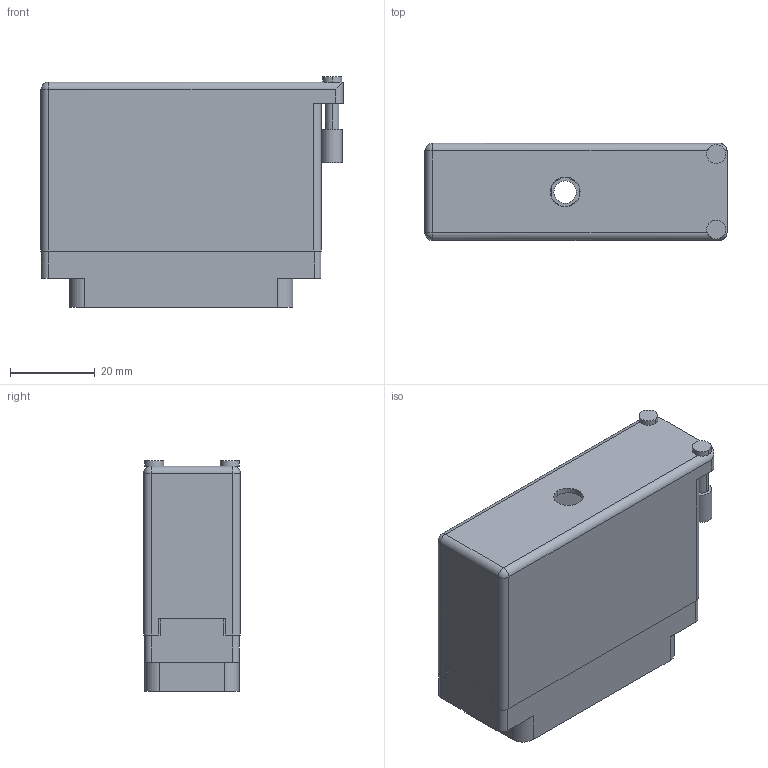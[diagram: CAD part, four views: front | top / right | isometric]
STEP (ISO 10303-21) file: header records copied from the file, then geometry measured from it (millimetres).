
FILE_DESCRIPTION (( 'STEP AP203' ), '1' );
FILE_NAME ('516-056-000-150.STEP', '2020-03-10T04:10:37', ( '' ), ( '' ), 'SwSTEP 2.0', 'SolidWorks 2016', '' );
FILE_SCHEMA (( 'CONFIG_CONTROL_DESIGN' ));
Length unit declared in the file: inch
Products named in the file (3): 516-056-000-150; 516 Plug Insulator_056; 516-230-001_Metal - 056 Side Entry
Assembly tree (2 placements, depth 2):
  516-056-000-150
    516 Plug Insulator_056
    516-230-001_Metal - 056 Side Entry
Bounding box: 71.12 x 22.83 x 54.31 mm (x, y, z)
Volume: 21855.5 mm3; surface area: 31798.8 mm2
Topology: 2 solids, 2 shells, 1280 faces, 3763 edges, 2502 vertices
Faces by surface type: plane 930, cylinder 346, cone 2, sphere 2
Entity records: 43134 total; most frequent: CARTESIAN_POINT 7589, ORIENTED_EDGE 7522, DIRECTION 7239, EDGE_CURVE 3761, LINE 2843, VECTOR 2843, VERTEX_POINT 2502, AXIS2_PLACEMENT_3D 2198
